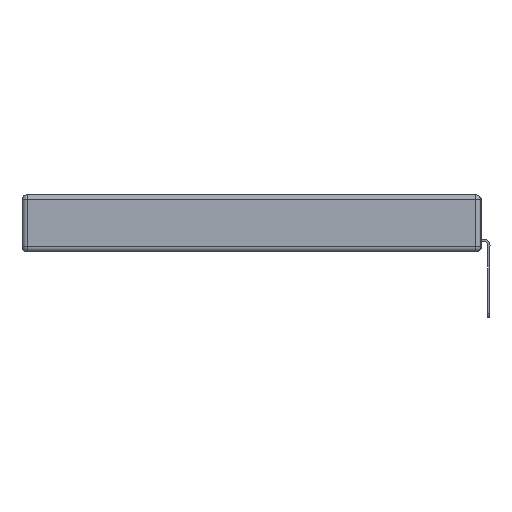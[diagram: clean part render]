
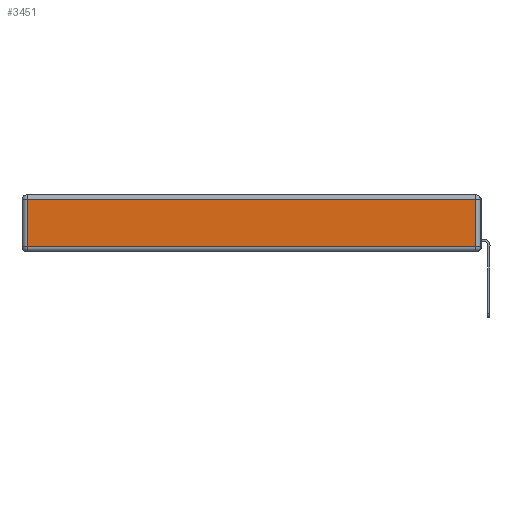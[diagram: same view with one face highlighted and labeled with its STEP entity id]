
A CAD part, left-side view. The second image highlights one B-rep face of the part: STEP entity #3451.
In plain terms, the highlighted planar face has unit normal (-1, 0, 0).
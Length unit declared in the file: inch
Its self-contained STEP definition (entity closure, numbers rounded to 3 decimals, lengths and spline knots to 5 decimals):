
#14 = EDGE_LOOP ( 'NONE', ( #5754, #21904, #3264, #14345 ) ) ;
#747 = LINE ( 'NONE', #841, #13276 ) ;
#841 = CARTESIAN_POINT ( 'NONE',  ( 0., 0.03, -0.343 ) ) ;
#1059 = DIRECTION ( 'NONE',  ( -1., 0., 0. ) ) ;
#1457 = CARTESIAN_POINT ( 'NONE',  ( 0., 2.72, -0.03 ) ) ;
#1713 = VERTEX_POINT ( 'NONE', #18600 ) ;
#2397 = LINE ( 'NONE', #16527, #2933 ) ;
#2710 = DIRECTION ( 'NONE',  ( 0., 0., 1. ) ) ;
#2933 = VECTOR ( 'NONE', #8150, 39.37008 ) ;
#3264 = ORIENTED_EDGE ( 'NONE', *, *, #20532, .T. ) ;
#3451 = ADVANCED_FACE ( 'NONE', ( #15973 ), #7790, .T. ) ;
#4493 = DIRECTION ( 'NONE',  ( 0., 0., 1. ) ) ;
#5443 = VERTEX_POINT ( 'NONE', #12895 ) ;
#5754 = ORIENTED_EDGE ( 'NONE', *, *, #14364, .T. ) ;
#5845 = VECTOR ( 'NONE', #5931, 39.37008 ) ;
#5931 = DIRECTION ( 'NONE',  ( 0., 0., -1. ) ) ;
#6101 = AXIS2_PLACEMENT_3D ( 'NONE', #18087, #1059, #4493 ) ;
#6612 = VECTOR ( 'NONE', #8262, 39.37008 ) ;
#6789 = VERTEX_POINT ( 'NONE', #10785 ) ;
#7790 = PLANE ( 'NONE',  #6101 ) ;
#8150 = DIRECTION ( 'NONE',  ( 0., -1., 0. ) ) ;
#8262 = DIRECTION ( 'NONE',  ( 0., 1., 0. ) ) ;
#10785 = CARTESIAN_POINT ( 'NONE',  ( 0., 0.03, -0.03 ) ) ;
#12895 = CARTESIAN_POINT ( 'NONE',  ( 0., 2.72, -0.313 ) ) ;
#13276 = VECTOR ( 'NONE', #2710, 39.37008 ) ;
#14345 = ORIENTED_EDGE ( 'NONE', *, *, #18083, .T. ) ;
#14364 = EDGE_CURVE ( 'NONE', #5443, #1713, #2397, .T. ) ;
#15364 = CARTESIAN_POINT ( 'NONE',  ( 0., 2.75, -0.03 ) ) ;
#15973 = FACE_OUTER_BOUND ( 'NONE', #14, .T. ) ;
#16527 = CARTESIAN_POINT ( 'NONE',  ( 0., 0., -0.313 ) ) ;
#18000 = CARTESIAN_POINT ( 'NONE',  ( 0., 2.72, -0.343 ) ) ;
#18066 = EDGE_CURVE ( 'NONE', #1713, #6789, #747, .T. ) ;
#18083 = EDGE_CURVE ( 'NONE', #20461, #5443, #18568, .T. ) ;
#18087 = CARTESIAN_POINT ( 'NONE',  ( 0., 0., -0.343 ) ) ;
#18568 = LINE ( 'NONE', #18000, #5845 ) ;
#18600 = CARTESIAN_POINT ( 'NONE',  ( 0., 0.03, -0.313 ) ) ;
#20461 = VERTEX_POINT ( 'NONE', #1457 ) ;
#20532 = EDGE_CURVE ( 'NONE', #6789, #20461, #21410, .T. ) ;
#21410 = LINE ( 'NONE', #15364, #6612 ) ;
#21904 = ORIENTED_EDGE ( 'NONE', *, *, #18066, .T. ) ;
